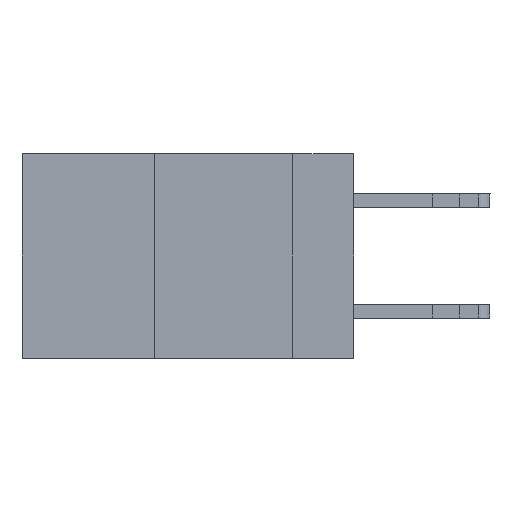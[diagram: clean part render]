
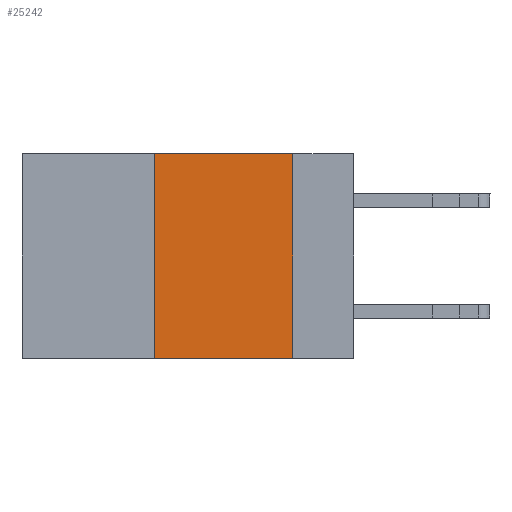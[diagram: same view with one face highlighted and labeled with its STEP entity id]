
A CAD part, left-side view. The second image highlights one B-rep face of the part: STEP entity #25242.
In plain terms, the highlighted planar face has unit normal (-1, 0, 0).
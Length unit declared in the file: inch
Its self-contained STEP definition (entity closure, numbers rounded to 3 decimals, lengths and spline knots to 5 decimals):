
#11 = VECTOR ( 'NONE', #18069, 39.37008 ) ;
#309 = EDGE_LOOP ( 'NONE', ( #14827, #10188, #39103, #11671 ) ) ;
#1015 = VECTOR ( 'NONE', #13352, 39.37008 ) ;
#1483 = VERTEX_POINT ( 'NONE', #7084 ) ;
#3996 = FACE_OUTER_BOUND ( 'NONE', #309, .T. ) ;
#4052 = CARTESIAN_POINT ( 'NONE',  ( 0., 0.36, 0. ) ) ;
#7084 = CARTESIAN_POINT ( 'NONE',  ( 0., 0.36, -0.37 ) ) ;
#7147 = DIRECTION ( 'NONE',  ( 1., 0., 0. ) ) ;
#8202 = DIRECTION ( 'NONE',  ( 0., 0., -1. ) ) ;
#9483 = VECTOR ( 'NONE', #8202, 39.37008 ) ;
#10188 = ORIENTED_EDGE ( 'NONE', *, *, #26375, .F. ) ;
#11006 = CARTESIAN_POINT ( 'NONE',  ( 0., 0.11, 0. ) ) ;
#11412 = LINE ( 'NONE', #11006, #9483 ) ;
#11671 = ORIENTED_EDGE ( 'NONE', *, *, #27956, .T. ) ;
#11755 = CARTESIAN_POINT ( 'NONE',  ( 0., 0.11, 0. ) ) ;
#12082 = EDGE_CURVE ( 'NONE', #1483, #33378, #18259, .T. ) ;
#13352 = DIRECTION ( 'NONE',  ( 0., -1., 0. ) ) ;
#14104 = CARTESIAN_POINT ( 'NONE',  ( 0., 0.6, -0.37 ) ) ;
#14827 = ORIENTED_EDGE ( 'NONE', *, *, #36968, .F. ) ;
#16931 = CARTESIAN_POINT ( 'NONE',  ( 0., 0.6, 0. ) ) ;
#17449 = AXIS2_PLACEMENT_3D ( 'NONE', #18894, #7147, #34069 ) ;
#18009 = CARTESIAN_POINT ( 'NONE',  ( 0., 0.11, -0.37 ) ) ;
#18069 = DIRECTION ( 'NONE',  ( 0., 0., 1. ) ) ;
#18229 = VECTOR ( 'NONE', #26272, 39.37008 ) ;
#18259 = LINE ( 'NONE', #33429, #11 ) ;
#18894 = CARTESIAN_POINT ( 'NONE',  ( 0., 0.6, 0. ) ) ;
#21891 = PLANE ( 'NONE',  #17449 ) ;
#25242 = ADVANCED_FACE ( 'NONE', ( #3996 ), #21891, .F. ) ;
#26272 = DIRECTION ( 'NONE',  ( 0., -1., 0. ) ) ;
#26375 = EDGE_CURVE ( 'NONE', #33378, #28856, #31486, .T. ) ;
#27956 = EDGE_CURVE ( 'NONE', #1483, #29872, #28665, .T. ) ;
#28665 = LINE ( 'NONE', #14104, #18229 ) ;
#28856 = VERTEX_POINT ( 'NONE', #11755 ) ;
#29872 = VERTEX_POINT ( 'NONE', #18009 ) ;
#31486 = LINE ( 'NONE', #16931, #1015 ) ;
#33378 = VERTEX_POINT ( 'NONE', #4052 ) ;
#33429 = CARTESIAN_POINT ( 'NONE',  ( 0., 0.36, 0. ) ) ;
#34069 = DIRECTION ( 'NONE',  ( 0., 0., -1. ) ) ;
#36968 = EDGE_CURVE ( 'NONE', #28856, #29872, #11412, .T. ) ;
#39103 = ORIENTED_EDGE ( 'NONE', *, *, #12082, .F. ) ;
